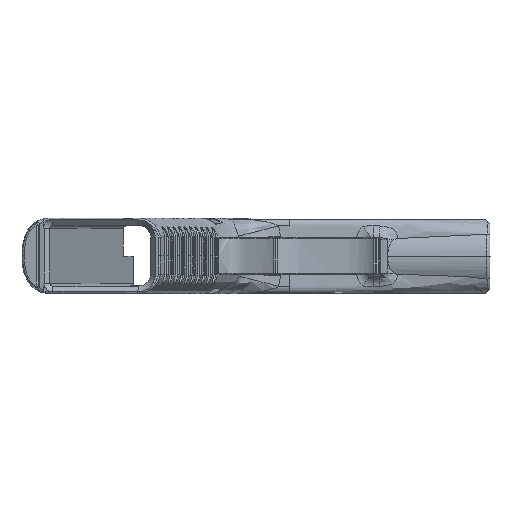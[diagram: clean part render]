
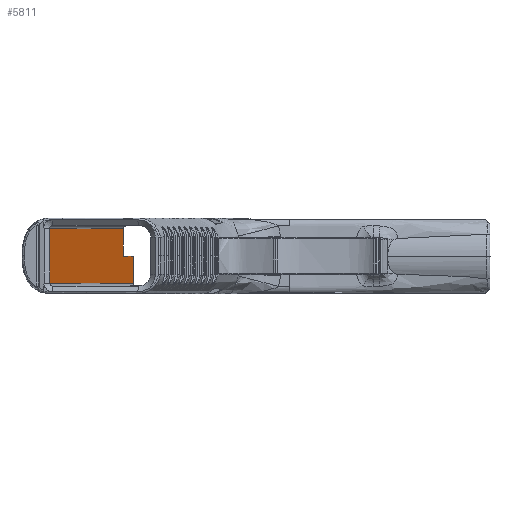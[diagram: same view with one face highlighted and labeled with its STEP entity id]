
A CAD part, top view. The second image highlights one B-rep face of the part: STEP entity #5811.
In plain terms, the highlighted planar face has unit normal (0.951, 0, 0.309).
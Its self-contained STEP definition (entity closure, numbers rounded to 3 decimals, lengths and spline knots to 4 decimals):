
#2272 = VECTOR ( 'NONE', #189524, 39.3701 ) ;
#5811 = ADVANCED_FACE ( 'NONE', ( #81074 ), #450859, .F. ) ;
#14153 = CARTESIAN_POINT ( 'NONE',  ( 2.0746, 0., -3.8765 ) ) ;
#54808 = LINE ( 'NONE', #146685, #398666 ) ;
#58366 = LINE ( 'NONE', #477633, #433206 ) ;
#63569 = CARTESIAN_POINT ( 'NONE',  ( 1.9466, 0., -3.4826 ) ) ;
#63919 = CARTESIAN_POINT ( 'NONE',  ( 2.0746, 0.0001, -3.8765 ) ) ;
#67923 = VECTOR ( 'NONE', #403316, 39.3701 ) ;
#81074 = FACE_OUTER_BOUND ( 'NONE', #125627, .T. ) ;
#125627 = EDGE_LOOP ( 'NONE', ( #453603, #155621, #295699, #393415, #372346, #261948 ) ) ;
#136576 = EDGE_CURVE ( 'NONE', #185738, #166118, #196164, .T. ) ;
#140385 = EDGE_CURVE ( 'NONE', #166118, #287165, #58366, .T. ) ;
#145601 = DIRECTION ( 'NONE',  ( 0., -1., 0. ) ) ;
#146685 = CARTESIAN_POINT ( 'NONE',  ( 2.0746, -0.37, -3.8765 ) ) ;
#155621 = ORIENTED_EDGE ( 'NONE', *, *, #140385, .F. ) ;
#166118 = VERTEX_POINT ( 'NONE', #415653 ) ;
#171382 = EDGE_CURVE ( 'NONE', #306124, #308691, #193191, .T. ) ;
#183660 = VECTOR ( 'NONE', #278628, 39.3701 ) ;
#185738 = VERTEX_POINT ( 'NONE', #250931 ) ;
#189524 = DIRECTION ( 'NONE',  ( 0.309, 0., -0.951 ) ) ;
#193191 = LINE ( 'NONE', #323021, #67923 ) ;
#193874 = CARTESIAN_POINT ( 'NONE',  ( 1.9466, 0.0001, -3.4826 ) ) ;
#194786 = CARTESIAN_POINT ( 'NONE',  ( 0.9499, 0., -0.4151 ) ) ;
#196164 = LINE ( 'NONE', #194786, #183660 ) ;
#209894 = DIRECTION ( 'NONE',  ( -0.309, 0., 0.951 ) ) ;
#220828 = LINE ( 'NONE', #63919, #2272 ) ;
#235640 = VECTOR ( 'NONE', #145601, 39.3701 ) ;
#241351 = AXIS2_PLACEMENT_3D ( 'NONE', #14153, #293696, #209894 ) ;
#249716 = CARTESIAN_POINT ( 'NONE',  ( 1.9466, 0.37, -3.4826 ) ) ;
#250931 = CARTESIAN_POINT ( 'NONE',  ( 0.9499, -0.37, -0.4151 ) ) ;
#261948 = ORIENTED_EDGE ( 'NONE', *, *, #432584, .F. ) ;
#278628 = DIRECTION ( 'NONE',  ( 0., 1., 0. ) ) ;
#287165 = VERTEX_POINT ( 'NONE', #249716 ) ;
#293696 = DIRECTION ( 'NONE',  ( -0.951, 0., -0.309 ) ) ;
#295699 = ORIENTED_EDGE ( 'NONE', *, *, #136576, .F. ) ;
#302568 = EDGE_CURVE ( 'NONE', #287165, #424403, #341938, .T. ) ;
#304823 = EDGE_CURVE ( 'NONE', #308691, #185738, #54808, .T. ) ;
#306124 = VERTEX_POINT ( 'NONE', #432376 ) ;
#308691 = VERTEX_POINT ( 'NONE', #406888 ) ;
#323021 = CARTESIAN_POINT ( 'NONE',  ( 2.0809, 0., -3.896 ) ) ;
#341938 = LINE ( 'NONE', #63569, #235640 ) ;
#372346 = ORIENTED_EDGE ( 'NONE', *, *, #171382, .F. ) ;
#393415 = ORIENTED_EDGE ( 'NONE', *, *, #304823, .F. ) ;
#398666 = VECTOR ( 'NONE', #508164, 39.3701 ) ;
#399049 = DIRECTION ( 'NONE',  ( 0.309, 0., -0.951 ) ) ;
#403316 = DIRECTION ( 'NONE',  ( 0., -1., 0. ) ) ;
#406888 = CARTESIAN_POINT ( 'NONE',  ( 2.0809, -0.37, -3.896 ) ) ;
#415653 = CARTESIAN_POINT ( 'NONE',  ( 0.9499, 0.37, -0.4151 ) ) ;
#424403 = VERTEX_POINT ( 'NONE', #193874 ) ;
#432376 = CARTESIAN_POINT ( 'NONE',  ( 2.0809, 0.0001, -3.896 ) ) ;
#432584 = EDGE_CURVE ( 'NONE', #424403, #306124, #220828, .T. ) ;
#433206 = VECTOR ( 'NONE', #399049, 39.3701 ) ;
#450859 = PLANE ( 'NONE',  #241351 ) ;
#453603 = ORIENTED_EDGE ( 'NONE', *, *, #302568, .F. ) ;
#477633 = CARTESIAN_POINT ( 'NONE',  ( 2.0746, 0.37, -3.8765 ) ) ;
#508164 = DIRECTION ( 'NONE',  ( -0.309, 0., 0.951 ) ) ;
